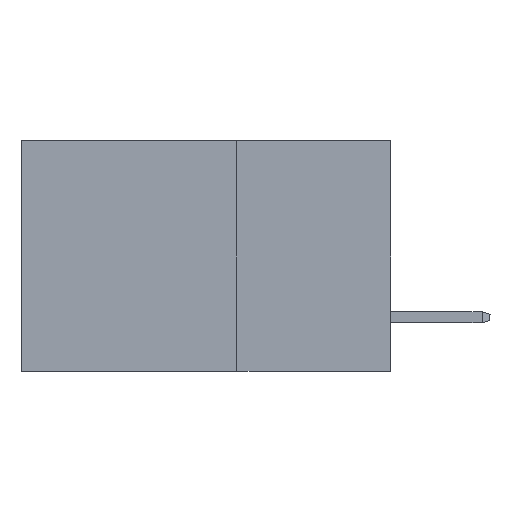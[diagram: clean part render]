
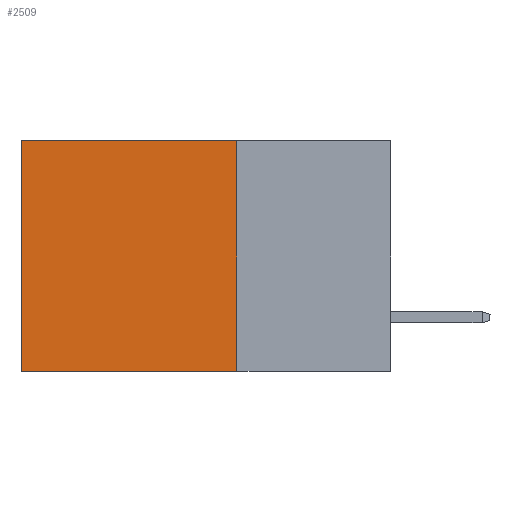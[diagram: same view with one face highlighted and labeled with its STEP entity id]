
A CAD part, left-side view. The second image highlights one B-rep face of the part: STEP entity #2509.
In plain terms, the highlighted planar face has unit normal (-1, 0, 0).
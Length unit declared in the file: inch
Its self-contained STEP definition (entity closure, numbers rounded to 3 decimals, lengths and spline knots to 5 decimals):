
#605 = DIRECTION ( 'NONE',  ( 0., 0., -1. ) ) ;
#702 = LINE ( 'NONE', #4779, #4214 ) ;
#931 = DIRECTION ( 'NONE',  ( 0., 1., 0. ) ) ;
#1031 = EDGE_CURVE ( 'NONE', #7723, #7779, #2208, .T. ) ;
#1378 = DIRECTION ( 'NONE',  ( 0., 0., -1. ) ) ;
#1626 = VERTEX_POINT ( 'NONE', #5205 ) ;
#2020 = EDGE_CURVE ( 'NONE', #1626, #7779, #6275, .T. ) ;
#2073 = FACE_OUTER_BOUND ( 'NONE', #6663, .T. ) ;
#2208 = LINE ( 'NONE', #6497, #7891 ) ;
#2312 = VECTOR ( 'NONE', #931, 39.37008 ) ;
#2380 = EDGE_CURVE ( 'NONE', #7200, #7723, #6952, .T. ) ;
#2432 = CARTESIAN_POINT ( 'NONE',  ( 0.2875, 0.6, 0. ) ) ;
#2509 = ADVANCED_FACE ( 'NONE', ( #2073 ), #5878, .F. ) ;
#2618 = DIRECTION ( 'NONE',  ( 0., 0., -1. ) ) ;
#2972 = DIRECTION ( 'NONE',  ( 1., 0., 0. ) ) ;
#4039 = CARTESIAN_POINT ( 'NONE',  ( 0.2875, 0.6, -0.375 ) ) ;
#4214 = VECTOR ( 'NONE', #2618, 39.37008 ) ;
#4528 = VECTOR ( 'NONE', #5719, 39.37008 ) ;
#4779 = CARTESIAN_POINT ( 'NONE',  ( 0.2875, 0.25, -0.375 ) ) ;
#5031 = CARTESIAN_POINT ( 'NONE',  ( 0.2875, 0.25, 0. ) ) ;
#5205 = CARTESIAN_POINT ( 'NONE',  ( 0.2875, 0.25, -0.375 ) ) ;
#5719 = DIRECTION ( 'NONE',  ( 0., 1., 0. ) ) ;
#5878 = PLANE ( 'NONE',  #9366 ) ;
#5975 = CARTESIAN_POINT ( 'NONE',  ( 0.2875, 0.25, -0.375 ) ) ;
#6207 = CARTESIAN_POINT ( 'NONE',  ( 0.2875, 0.25, -0.375 ) ) ;
#6275 = LINE ( 'NONE', #6207, #2312 ) ;
#6497 = CARTESIAN_POINT ( 'NONE',  ( 0.2875, 0.6, -0.375 ) ) ;
#6663 = EDGE_LOOP ( 'NONE', ( #8145, #7281, #7444, #8127 ) ) ;
#6771 = EDGE_CURVE ( 'NONE', #7200, #1626, #702, .T. ) ;
#6952 = LINE ( 'NONE', #5031, #4528 ) ;
#7200 = VERTEX_POINT ( 'NONE', #7728 ) ;
#7281 = ORIENTED_EDGE ( 'NONE', *, *, #2020, .F. ) ;
#7444 = ORIENTED_EDGE ( 'NONE', *, *, #6771, .F. ) ;
#7723 = VERTEX_POINT ( 'NONE', #2432 ) ;
#7728 = CARTESIAN_POINT ( 'NONE',  ( 0.2875, 0.25, 0. ) ) ;
#7779 = VERTEX_POINT ( 'NONE', #4039 ) ;
#7891 = VECTOR ( 'NONE', #605, 39.37008 ) ;
#8127 = ORIENTED_EDGE ( 'NONE', *, *, #2380, .T. ) ;
#8145 = ORIENTED_EDGE ( 'NONE', *, *, #1031, .T. ) ;
#9366 = AXIS2_PLACEMENT_3D ( 'NONE', #5975, #2972, #1378 ) ;
